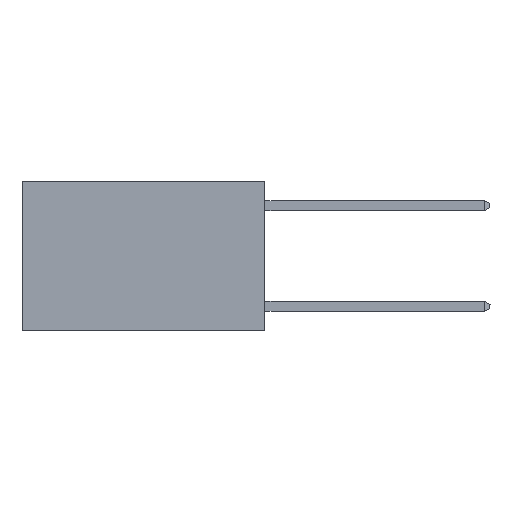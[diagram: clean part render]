
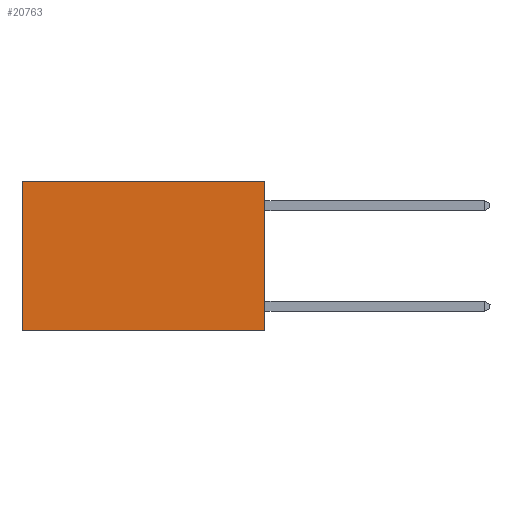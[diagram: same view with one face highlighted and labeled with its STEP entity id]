
A CAD part, left-side view. The second image highlights one B-rep face of the part: STEP entity #20763.
In plain terms, the highlighted planar face has unit normal (-1, 0, 0).
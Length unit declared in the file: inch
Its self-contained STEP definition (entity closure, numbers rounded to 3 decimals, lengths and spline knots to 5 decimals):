
#58 = PLANE ( 'NONE',  #17901 ) ;
#141 = DIRECTION ( 'NONE',  ( 0., 0., -1. ) ) ;
#1609 = LINE ( 'NONE', #7850, #20891 ) ;
#2193 = VECTOR ( 'NONE', #21668, 39.37008 ) ;
#2263 = CARTESIAN_POINT ( 'NONE',  ( 0.2625, 0., -0.37 ) ) ;
#2998 = CARTESIAN_POINT ( 'NONE',  ( 0.2625, 0., 0. ) ) ;
#3869 = ORIENTED_EDGE ( 'NONE', *, *, #6915, .T. ) ;
#5389 = EDGE_CURVE ( 'NONE', #13540, #11423, #22014, .T. ) ;
#5961 = FACE_OUTER_BOUND ( 'NONE', #17769, .T. ) ;
#6057 = DIRECTION ( 'NONE',  ( 0., 0., -1. ) ) ;
#6164 = ORIENTED_EDGE ( 'NONE', *, *, #11068, .F. ) ;
#6215 = DIRECTION ( 'NONE',  ( 0., 0., -1. ) ) ;
#6414 = EDGE_CURVE ( 'NONE', #9662, #19561, #13588, .T. ) ;
#6915 = EDGE_CURVE ( 'NONE', #11423, #19561, #22818, .T. ) ;
#7591 = CARTESIAN_POINT ( 'NONE',  ( 0.2625, 0., 0. ) ) ;
#7850 = CARTESIAN_POINT ( 'NONE',  ( 0.2625, 0., 0. ) ) ;
#7974 = VECTOR ( 'NONE', #6215, 39.37008 ) ;
#9662 = VERTEX_POINT ( 'NONE', #2263 ) ;
#9993 = CARTESIAN_POINT ( 'NONE',  ( 0.2625, 0.6, 0. ) ) ;
#10140 = ORIENTED_EDGE ( 'NONE', *, *, #5389, .T. ) ;
#11068 = EDGE_CURVE ( 'NONE', #13540, #9662, #1609, .T. ) ;
#11333 = DIRECTION ( 'NONE',  ( 1., 0., 0. ) ) ;
#11423 = VERTEX_POINT ( 'NONE', #18260 ) ;
#11809 = CARTESIAN_POINT ( 'NONE',  ( 0.2625, 0.6, -0.37 ) ) ;
#13540 = VERTEX_POINT ( 'NONE', #15283 ) ;
#13588 = LINE ( 'NONE', #21628, #15319 ) ;
#15283 = CARTESIAN_POINT ( 'NONE',  ( 0.2625, 0., 0. ) ) ;
#15319 = VECTOR ( 'NONE', #19825, 39.37008 ) ;
#17769 = EDGE_LOOP ( 'NONE', ( #3869, #20791, #6164, #10140 ) ) ;
#17901 = AXIS2_PLACEMENT_3D ( 'NONE', #7591, #11333, #141 ) ;
#18260 = CARTESIAN_POINT ( 'NONE',  ( 0.2625, 0.6, 0. ) ) ;
#19561 = VERTEX_POINT ( 'NONE', #11809 ) ;
#19825 = DIRECTION ( 'NONE',  ( 0., 1., 0. ) ) ;
#20763 = ADVANCED_FACE ( 'NONE', ( #5961 ), #58, .F. ) ;
#20791 = ORIENTED_EDGE ( 'NONE', *, *, #6414, .F. ) ;
#20891 = VECTOR ( 'NONE', #6057, 39.37008 ) ;
#21628 = CARTESIAN_POINT ( 'NONE',  ( 0.2625, 0., -0.37 ) ) ;
#21668 = DIRECTION ( 'NONE',  ( 0., 1., 0. ) ) ;
#22014 = LINE ( 'NONE', #2998, #2193 ) ;
#22818 = LINE ( 'NONE', #9993, #7974 ) ;
